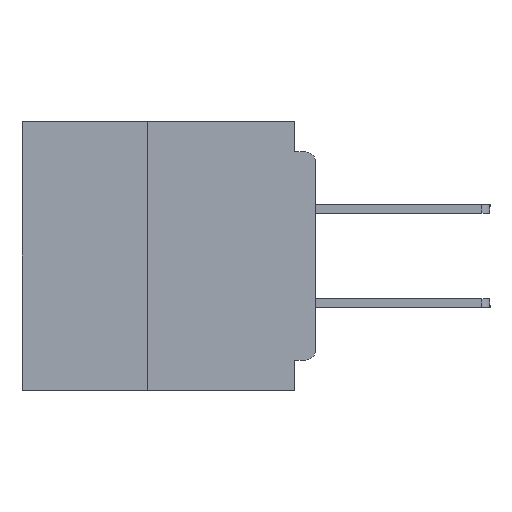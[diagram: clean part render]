
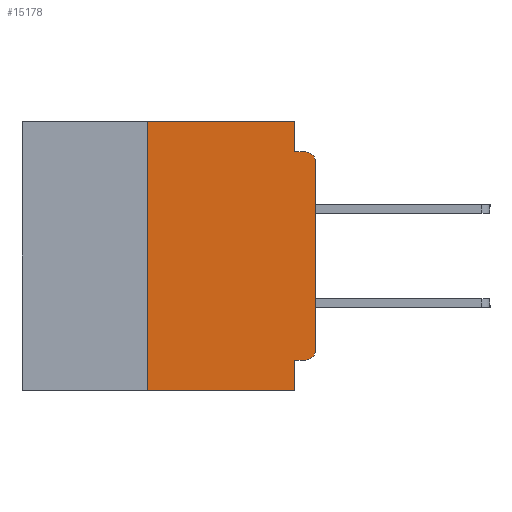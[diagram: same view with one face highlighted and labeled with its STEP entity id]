
A CAD part, left-side view. The second image highlights one B-rep face of the part: STEP entity #15178.
In plain terms, the highlighted planar face has unit normal (-1, 0, 0).
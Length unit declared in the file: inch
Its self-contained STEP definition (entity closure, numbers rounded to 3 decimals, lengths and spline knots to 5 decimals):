
#562 = ORIENTED_EDGE ( 'NONE', *, *, #51108, .F. ) ;
#866 = EDGE_CURVE ( 'NONE', #18206, #15473, #24548, .T. ) ;
#1802 = DIRECTION ( 'NONE',  ( 0., -1., 0. ) ) ;
#2109 = CARTESIAN_POINT ( 'NONE',  ( 0., 0.031, 0. ) ) ;
#2137 = CARTESIAN_POINT ( 'NONE',  ( 0., 0., -0.06 ) ) ;
#2415 = EDGE_CURVE ( 'NONE', #14205, #60600, #7869, .T. ) ;
#2542 = LINE ( 'NONE', #45461, #51166 ) ;
#3398 = CARTESIAN_POINT ( 'NONE',  ( 0., 0.25, 0. ) ) ;
#3696 = VERTEX_POINT ( 'NONE', #7232 ) ;
#3808 = EDGE_CURVE ( 'NONE', #60925, #13637, #33575, .T. ) ;
#4653 = DIRECTION ( 'NONE',  ( 1., 0., 0. ) ) ;
#5333 = ORIENTED_EDGE ( 'NONE', *, *, #866, .T. ) ;
#5467 = CARTESIAN_POINT ( 'NONE',  ( 0., 0.015, -0.355 ) ) ;
#7130 = AXIS2_PLACEMENT_3D ( 'NONE', #38830, #10586, #43502 ) ;
#7232 = CARTESIAN_POINT ( 'NONE',  ( 0., 0.015, -0.045 ) ) ;
#7869 = LINE ( 'NONE', #20547, #31424 ) ;
#8067 = DIRECTION ( 'NONE',  ( 0., 1., 0. ) ) ;
#10308 = VECTOR ( 'NONE', #48314, 39.37008 ) ;
#10586 = DIRECTION ( 'NONE',  ( -1., 0., 0. ) ) ;
#10920 = AXIS2_PLACEMENT_3D ( 'NONE', #18660, #4653, #37633 ) ;
#10938 = ORIENTED_EDGE ( 'NONE', *, *, #33091, .T. ) ;
#11219 = CARTESIAN_POINT ( 'NONE',  ( 0., 0.031, -0.355 ) ) ;
#12058 = VECTOR ( 'NONE', #32086, 39.37008 ) ;
#13637 = VERTEX_POINT ( 'NONE', #11219 ) ;
#13829 = ORIENTED_EDGE ( 'NONE', *, *, #34626, .F. ) ;
#14205 = VERTEX_POINT ( 'NONE', #24719 ) ;
#14477 = CARTESIAN_POINT ( 'NONE',  ( 0., 0., -0.045 ) ) ;
#15178 = ADVANCED_FACE ( 'NONE', ( #47684 ), #32885, .F. ) ;
#15473 = VERTEX_POINT ( 'NONE', #2137 ) ;
#18206 = VERTEX_POINT ( 'NONE', #51315 ) ;
#18660 = CARTESIAN_POINT ( 'NONE',  ( 0., 0.437, 0. ) ) ;
#20547 = CARTESIAN_POINT ( 'NONE',  ( 0., 0.437, -0.4 ) ) ;
#21792 = DIRECTION ( 'NONE',  ( 0., 0., 1. ) ) ;
#22828 = LINE ( 'NONE', #57536, #10308 ) ;
#23228 = DIRECTION ( 'NONE',  ( -1., 0., 0. ) ) ;
#23683 = AXIS2_PLACEMENT_3D ( 'NONE', #51414, #23228, #56075 ) ;
#24217 = LINE ( 'NONE', #2109, #60249 ) ;
#24548 = LINE ( 'NONE', #42635, #12058 ) ;
#24719 = CARTESIAN_POINT ( 'NONE',  ( 0., 0.25, -0.4 ) ) ;
#27123 = ORIENTED_EDGE ( 'NONE', *, *, #29241, .F. ) ;
#29241 = EDGE_CURVE ( 'NONE', #36160, #3696, #31710, .T. ) ;
#31424 = VECTOR ( 'NONE', #1802, 39.37008 ) ;
#31710 = LINE ( 'NONE', #14477, #55200 ) ;
#32086 = DIRECTION ( 'NONE',  ( 0., 0., 1. ) ) ;
#32884 = VERTEX_POINT ( 'NONE', #3398 ) ;
#32885 = PLANE ( 'NONE',  #10920 ) ;
#32958 = CARTESIAN_POINT ( 'NONE',  ( 0., 0.031, -0.045 ) ) ;
#33091 = EDGE_CURVE ( 'NONE', #60925, #18206, #44364, .T. ) ;
#33575 = LINE ( 'NONE', #50235, #55577 ) ;
#34527 = EDGE_CURVE ( 'NONE', #13637, #60600, #22828, .T. ) ;
#34626 = EDGE_CURVE ( 'NONE', #14205, #32884, #41986, .T. ) ;
#35317 = ORIENTED_EDGE ( 'NONE', *, *, #3808, .F. ) ;
#36160 = VERTEX_POINT ( 'NONE', #32958 ) ;
#37633 = DIRECTION ( 'NONE',  ( 0., 0., -1. ) ) ;
#37935 = CIRCLE ( 'NONE', #23683, 0.015 ) ;
#38830 = CARTESIAN_POINT ( 'NONE',  ( 0., 0.015, -0.34 ) ) ;
#39630 = DIRECTION ( 'NONE',  ( 0., 0., -1. ) ) ;
#41269 = ORIENTED_EDGE ( 'NONE', *, *, #2415, .T. ) ;
#41986 = LINE ( 'NONE', #49977, #52965 ) ;
#42635 = CARTESIAN_POINT ( 'NONE',  ( 0., 0., 0. ) ) ;
#42660 = DIRECTION ( 'NONE',  ( 0., -1., 0. ) ) ;
#43502 = DIRECTION ( 'NONE',  ( 0., 0., -1. ) ) ;
#44364 = CIRCLE ( 'NONE', #7130, 0.015 ) ;
#45461 = CARTESIAN_POINT ( 'NONE',  ( 0., 0.437, 0. ) ) ;
#45649 = CARTESIAN_POINT ( 'NONE',  ( 0., 0.031, -0.4 ) ) ;
#46768 = EDGE_LOOP ( 'NONE', ( #5333, #46975, #27123, #562, #52623, #13829, #41269, #48556, #35317, #10938 ) ) ;
#46975 = ORIENTED_EDGE ( 'NONE', *, *, #48911, .T. ) ;
#47684 = FACE_OUTER_BOUND ( 'NONE', #46768, .T. ) ;
#48314 = DIRECTION ( 'NONE',  ( 0., 0., -1. ) ) ;
#48556 = ORIENTED_EDGE ( 'NONE', *, *, #34527, .F. ) ;
#48911 = EDGE_CURVE ( 'NONE', #15473, #3696, #37935, .T. ) ;
#49977 = CARTESIAN_POINT ( 'NONE',  ( 0., 0.25, -0.4 ) ) ;
#50181 = DIRECTION ( 'NONE',  ( 0., -1., 0. ) ) ;
#50235 = CARTESIAN_POINT ( 'NONE',  ( 0., 0., -0.355 ) ) ;
#51108 = EDGE_CURVE ( 'NONE', #52293, #36160, #24217, .T. ) ;
#51166 = VECTOR ( 'NONE', #50181, 39.37008 ) ;
#51315 = CARTESIAN_POINT ( 'NONE',  ( 0., 0., -0.34 ) ) ;
#51414 = CARTESIAN_POINT ( 'NONE',  ( 0., 0.015, -0.06 ) ) ;
#52293 = VERTEX_POINT ( 'NONE', #58948 ) ;
#52623 = ORIENTED_EDGE ( 'NONE', *, *, #59516, .F. ) ;
#52965 = VECTOR ( 'NONE', #21792, 39.37008 ) ;
#55200 = VECTOR ( 'NONE', #42660, 39.37008 ) ;
#55577 = VECTOR ( 'NONE', #8067, 39.37008 ) ;
#56075 = DIRECTION ( 'NONE',  ( 0., 0., -1. ) ) ;
#57536 = CARTESIAN_POINT ( 'NONE',  ( 0., 0.031, -0.4 ) ) ;
#58948 = CARTESIAN_POINT ( 'NONE',  ( 0., 0.031, 0. ) ) ;
#59516 = EDGE_CURVE ( 'NONE', #32884, #52293, #2542, .T. ) ;
#60249 = VECTOR ( 'NONE', #39630, 39.37008 ) ;
#60600 = VERTEX_POINT ( 'NONE', #45649 ) ;
#60925 = VERTEX_POINT ( 'NONE', #5467 ) ;
